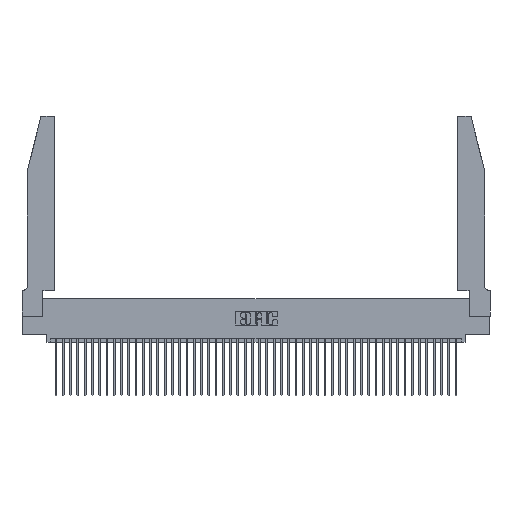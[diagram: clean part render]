
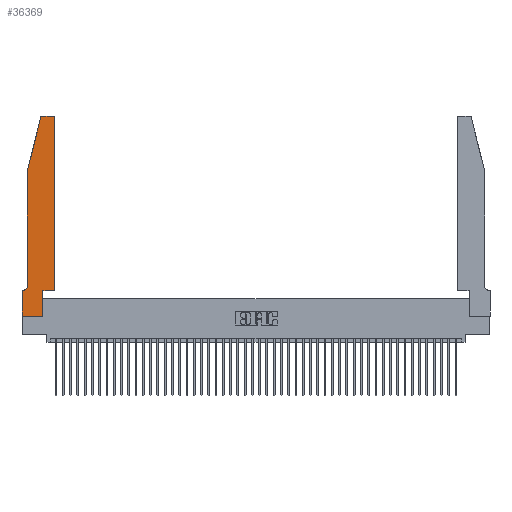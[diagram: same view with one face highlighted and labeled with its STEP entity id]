
A CAD part, top view. The second image highlights one B-rep face of the part: STEP entity #36369.
In plain terms, the highlighted planar face has unit normal (0, 0, 1).
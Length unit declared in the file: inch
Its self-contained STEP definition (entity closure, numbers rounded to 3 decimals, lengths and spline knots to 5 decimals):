
#149 = LINE ( 'NONE', #32379, #18445 ) ;
#370 = DIRECTION ( 'NONE',  ( 1., 0., 0. ) ) ;
#519 = CARTESIAN_POINT ( 'NONE',  ( 0.4205, 2.75, 0.37 ) ) ;
#683 = EDGE_CURVE ( 'NONE', #40575, #9690, #149, .T. ) ;
#3491 = VERTEX_POINT ( 'NONE', #4975 ) ;
#3504 = EDGE_CURVE ( 'NONE', #38094, #18149, #44738, .T. ) ;
#4652 = DIRECTION ( 'NONE',  ( 1., 0., 0. ) ) ;
#4863 = ORIENTED_EDGE ( 'NONE', *, *, #42003, .T. ) ;
#4975 = CARTESIAN_POINT ( 'NONE',  ( 0.0755, 0.42, 0.37 ) ) ;
#5040 = DIRECTION ( 'NONE',  ( -1., 0., 0. ) ) ;
#5453 = CARTESIAN_POINT ( 'NONE',  ( 0.284, 2.72, 0.37 ) ) ;
#5887 = CIRCLE ( 'NONE', #33764, 0.03 ) ;
#6539 = VERTEX_POINT ( 'NONE', #33968 ) ;
#8795 = DIRECTION ( 'NONE',  ( 0., 0., 1. ) ) ;
#9112 = DIRECTION ( 'NONE',  ( 1., 0., 0. ) ) ;
#9261 = CARTESIAN_POINT ( 'NONE',  ( 0., 0., 0.37 ) ) ;
#9440 = ORIENTED_EDGE ( 'NONE', *, *, #17549, .T. ) ;
#9690 = VERTEX_POINT ( 'NONE', #40053 ) ;
#10980 = DIRECTION ( 'NONE',  ( 1., 0., 0. ) ) ;
#11596 = CARTESIAN_POINT ( 'NONE',  ( 0.4505, 2.72, 0.37 ) ) ;
#11696 = ORIENTED_EDGE ( 'NONE', *, *, #18374, .T. ) ;
#11715 = CARTESIAN_POINT ( 'NONE',  ( 0.2865, 0.35, 0.37 ) ) ;
#11887 = DIRECTION ( 'NONE',  ( 0., 1., 0. ) ) ;
#12882 = VERTEX_POINT ( 'NONE', #11715 ) ;
#13104 = CARTESIAN_POINT ( 'NONE',  ( 0.0055, 0.35, 0.37 ) ) ;
#13501 = VERTEX_POINT ( 'NONE', #45260 ) ;
#14314 = LINE ( 'NONE', #44443, #32494 ) ;
#14417 = FACE_OUTER_BOUND ( 'NONE', #32491, .T. ) ;
#14779 = CARTESIAN_POINT ( 'NONE',  ( 0.0755, 0.35, 0.37 ) ) ;
#14911 = PLANE ( 'NONE',  #19483 ) ;
#15172 = EDGE_CURVE ( 'NONE', #23041, #12882, #31123, .T. ) ;
#15338 = ORIENTED_EDGE ( 'NONE', *, *, #683, .T. ) ;
#15574 = CARTESIAN_POINT ( 'NONE',  ( 0.2865, 0.35, 0.37 ) ) ;
#16631 = ORIENTED_EDGE ( 'NONE', *, *, #22415, .T. ) ;
#16663 = LINE ( 'NONE', #14779, #44381 ) ;
#17453 = ORIENTED_EDGE ( 'NONE', *, *, #26424, .T. ) ;
#17549 = EDGE_CURVE ( 'NONE', #42766, #23337, #16663, .T. ) ;
#18081 = CARTESIAN_POINT ( 'NONE',  ( 0.25487, 2.72718, 0.37 ) ) ;
#18149 = VERTEX_POINT ( 'NONE', #519 ) ;
#18374 = EDGE_CURVE ( 'NONE', #23337, #6539, #30809, .T. ) ;
#18445 = VECTOR ( 'NONE', #28729, 39.37008 ) ;
#18596 = CARTESIAN_POINT ( 'NONE',  ( 0., 0.35, 0.37 ) ) ;
#19198 = ORIENTED_EDGE ( 'NONE', *, *, #39325, .T. ) ;
#19483 = AXIS2_PLACEMENT_3D ( 'NONE', #18596, #22229, #370 ) ;
#19587 = CARTESIAN_POINT ( 'NONE',  ( 0.2605, 2.75, 0.37 ) ) ;
#19771 = DIRECTION ( 'NONE',  ( 0., 0., -1. ) ) ;
#20040 = DIRECTION ( 'NONE',  ( 0., -1., 0. ) ) ;
#20306 = DIRECTION ( 'NONE',  ( 0., -1., 0. ) ) ;
#20876 = VECTOR ( 'NONE', #20040, 39.37008 ) ;
#21291 = LINE ( 'NONE', #32808, #32067 ) ;
#21498 = ORIENTED_EDGE ( 'NONE', *, *, #15172, .T. ) ;
#22229 = DIRECTION ( 'NONE',  ( 0., 0., 1. ) ) ;
#22415 = EDGE_CURVE ( 'NONE', #13501, #38094, #46003, .T. ) ;
#23041 = VERTEX_POINT ( 'NONE', #32097 ) ;
#23337 = VERTEX_POINT ( 'NONE', #37429 ) ;
#24721 = ORIENTED_EDGE ( 'NONE', *, *, #3504, .T. ) ;
#25073 = CARTESIAN_POINT ( 'NONE',  ( 0.284, 2.75, 0.37 ) ) ;
#25886 = VECTOR ( 'NONE', #5040, 39.37008 ) ;
#26107 = EDGE_CURVE ( 'NONE', #46793, #40575, #5887, .T. ) ;
#26424 = EDGE_CURVE ( 'NONE', #12882, #13501, #21291, .T. ) ;
#26680 = AXIS2_PLACEMENT_3D ( 'NONE', #30605, #8795, #34219 ) ;
#26866 = VECTOR ( 'NONE', #32623, 39.37008 ) ;
#26870 = ORIENTED_EDGE ( 'NONE', *, *, #26107, .T. ) ;
#26901 = AXIS2_PLACEMENT_3D ( 'NONE', #41354, #19771, #44982 ) ;
#28729 = DIRECTION ( 'NONE',  ( -0.239, -0.971, 0. ) ) ;
#30524 = LINE ( 'NONE', #38055, #20876 ) ;
#30543 = CIRCLE ( 'NONE', #26901, 0.07 ) ;
#30605 = CARTESIAN_POINT ( 'NONE',  ( 0.4205, 2.72, 0.37 ) ) ;
#30607 = EDGE_CURVE ( 'NONE', #3491, #42766, #30543, .T. ) ;
#30809 = LINE ( 'NONE', #9261, #40362 ) ;
#30938 = DIRECTION ( 'NONE',  ( 0., 0., 1. ) ) ;
#31123 = LINE ( 'NONE', #15574, #39543 ) ;
#32067 = VECTOR ( 'NONE', #10980, 39.37008 ) ;
#32097 = CARTESIAN_POINT ( 'NONE',  ( 0.2865, 0., 0.37 ) ) ;
#32379 = CARTESIAN_POINT ( 'NONE',  ( 0.0755, 2., 0.37 ) ) ;
#32491 = EDGE_LOOP ( 'NONE', ( #38003, #26870, #15338, #4863, #40259, #9440, #11696, #19198, #21498, #17453, #16631, #24721 ) ) ;
#32494 = VECTOR ( 'NONE', #4652, 39.37008 ) ;
#32623 = DIRECTION ( 'NONE',  ( 0., 1., 0. ) ) ;
#32808 = CARTESIAN_POINT ( 'NONE',  ( 0.4505, 0.35, 0.37 ) ) ;
#33764 = AXIS2_PLACEMENT_3D ( 'NONE', #5453, #30938, #9112 ) ;
#33968 = CARTESIAN_POINT ( 'NONE',  ( 0., 0., 0.37 ) ) ;
#34219 = DIRECTION ( 'NONE',  ( 1., 0., 0. ) ) ;
#35482 = LINE ( 'NONE', #19587, #25886 ) ;
#36369 = ADVANCED_FACE ( 'NONE', ( #14417 ), #14911, .T. ) ;
#37429 = CARTESIAN_POINT ( 'NONE',  ( 0., 0.35, 0.37 ) ) ;
#38003 = ORIENTED_EDGE ( 'NONE', *, *, #43434, .T. ) ;
#38055 = CARTESIAN_POINT ( 'NONE',  ( 0.0755, 2., 0.37 ) ) ;
#38094 = VERTEX_POINT ( 'NONE', #11596 ) ;
#39325 = EDGE_CURVE ( 'NONE', #6539, #23041, #14314, .T. ) ;
#39543 = VECTOR ( 'NONE', #11887, 39.37008 ) ;
#40053 = CARTESIAN_POINT ( 'NONE',  ( 0.0755, 2., 0.37 ) ) ;
#40259 = ORIENTED_EDGE ( 'NONE', *, *, #30607, .T. ) ;
#40362 = VECTOR ( 'NONE', #20306, 39.37008 ) ;
#40575 = VERTEX_POINT ( 'NONE', #18081 ) ;
#41354 = CARTESIAN_POINT ( 'NONE',  ( 0.0055, 0.42, 0.37 ) ) ;
#42003 = EDGE_CURVE ( 'NONE', #9690, #3491, #30524, .T. ) ;
#42766 = VERTEX_POINT ( 'NONE', #13104 ) ;
#43434 = EDGE_CURVE ( 'NONE', #18149, #46793, #35482, .T. ) ;
#43705 = DIRECTION ( 'NONE',  ( -1., 0., 0. ) ) ;
#44381 = VECTOR ( 'NONE', #43705, 39.37008 ) ;
#44443 = CARTESIAN_POINT ( 'NONE',  ( 0., 0., 0.37 ) ) ;
#44738 = CIRCLE ( 'NONE', #26680, 0.03 ) ;
#44982 = DIRECTION ( 'NONE',  ( -1., 0., 0. ) ) ;
#45260 = CARTESIAN_POINT ( 'NONE',  ( 0.4505, 0.35, 0.37 ) ) ;
#46003 = LINE ( 'NONE', #46922, #26866 ) ;
#46793 = VERTEX_POINT ( 'NONE', #25073 ) ;
#46922 = CARTESIAN_POINT ( 'NONE',  ( 0.4505, 0.35, 0.37 ) ) ;
